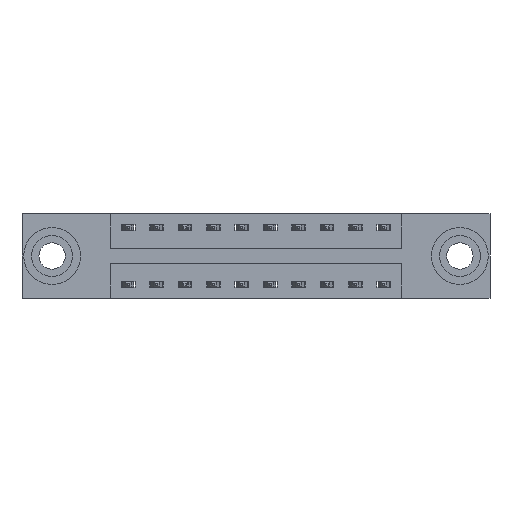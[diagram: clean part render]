
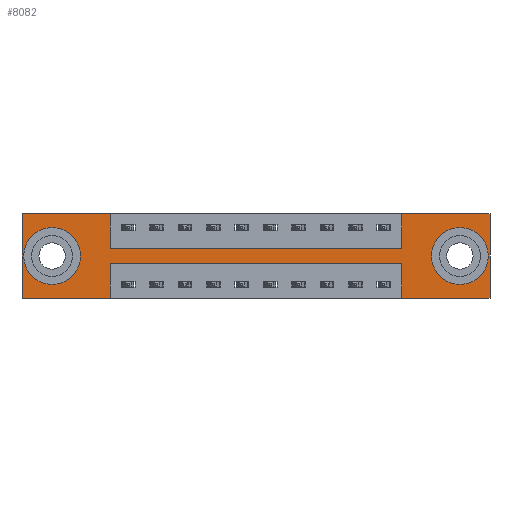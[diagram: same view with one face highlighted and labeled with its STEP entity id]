
A CAD part, front view. The second image highlights one B-rep face of the part: STEP entity #8082.
In plain terms, the highlighted planar face has unit normal (0, -1, 0).
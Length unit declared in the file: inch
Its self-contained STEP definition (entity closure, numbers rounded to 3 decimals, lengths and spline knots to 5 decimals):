
#42 = DIRECTION ( 'NONE',  ( 0., -1., 0. ) ) ;
#43 = FACE_BOUND ( 'NONE', #593, .T. ) ;
#147 = VECTOR ( 'NONE', #8115, 39.37008 ) ;
#241 = VERTEX_POINT ( 'NONE', #6588 ) ;
#277 = LINE ( 'NONE', #2341, #9574 ) ;
#318 = ORIENTED_EDGE ( 'NONE', *, *, #9186, .F. ) ;
#549 = LINE ( 'NONE', #3634, #4817 ) ;
#587 = CARTESIAN_POINT ( 'NONE',  ( 0.1325, 0., -0.107 ) ) ;
#593 = EDGE_LOOP ( 'NONE', ( #3263, #9373 ) ) ;
#647 = VERTEX_POINT ( 'NONE', #587 ) ;
#715 = ORIENTED_EDGE ( 'NONE', *, *, #3918, .F. ) ;
#737 = EDGE_CURVE ( 'NONE', #647, #7364, #2487, .T. ) ;
#756 = CARTESIAN_POINT ( 'NONE',  ( 2.06, 0., 0. ) ) ;
#1233 = ORIENTED_EDGE ( 'NONE', *, *, #1397, .F. ) ;
#1290 = VECTOR ( 'NONE', #8873, 39.37008 ) ;
#1392 = CARTESIAN_POINT ( 'NONE',  ( 1.9275, 0., -0.185 ) ) ;
#1397 = EDGE_CURVE ( 'NONE', #10675, #7529, #8215, .T. ) ;
#1768 = LINE ( 'NONE', #4602, #6515 ) ;
#1775 = VERTEX_POINT ( 'NONE', #10320 ) ;
#1825 = CARTESIAN_POINT ( 'NONE',  ( 0.1325, 0., -0.263 ) ) ;
#1854 = DIRECTION ( 'NONE',  ( 0., 0., -1. ) ) ;
#1980 = VECTOR ( 'NONE', #3044, 39.37008 ) ;
#1993 = EDGE_CURVE ( 'NONE', #7529, #5907, #9125, .T. ) ;
#2018 = CARTESIAN_POINT ( 'NONE',  ( 1.6725, 0., 0. ) ) ;
#2274 = DIRECTION ( 'NONE',  ( 0., 0., -1. ) ) ;
#2341 = CARTESIAN_POINT ( 'NONE',  ( 1.6725, 0., -0.37 ) ) ;
#2402 = VERTEX_POINT ( 'NONE', #4442 ) ;
#2419 = DIRECTION ( 'NONE',  ( 1., 0., 0. ) ) ;
#2438 = ORIENTED_EDGE ( 'NONE', *, *, #6224, .F. ) ;
#2453 = AXIS2_PLACEMENT_3D ( 'NONE', #4191, #8225, #9523 ) ;
#2487 = CIRCLE ( 'NONE', #2453, 0.078 ) ;
#2491 = DIRECTION ( 'NONE',  ( 0., 1., 0. ) ) ;
#2676 = CARTESIAN_POINT ( 'NONE',  ( 0.3875, 0., -0.22 ) ) ;
#2740 = CARTESIAN_POINT ( 'NONE',  ( 0., 0., -0.37 ) ) ;
#2778 = DIRECTION ( 'NONE',  ( 1., 0., 0. ) ) ;
#3044 = DIRECTION ( 'NONE',  ( -1., 0., 0. ) ) ;
#3046 = VERTEX_POINT ( 'NONE', #3427 ) ;
#3263 = ORIENTED_EDGE ( 'NONE', *, *, #737, .T. ) ;
#3427 = CARTESIAN_POINT ( 'NONE',  ( 1.6725, 0., -0.22 ) ) ;
#3443 = CARTESIAN_POINT ( 'NONE',  ( 1.9275, 0., -0.185 ) ) ;
#3548 = EDGE_CURVE ( 'NONE', #7974, #2402, #10690, .T. ) ;
#3634 = CARTESIAN_POINT ( 'NONE',  ( 0.3875, 0., 0. ) ) ;
#3750 = EDGE_CURVE ( 'NONE', #7364, #647, #6431, .T. ) ;
#3839 = VERTEX_POINT ( 'NONE', #7047 ) ;
#3918 = EDGE_CURVE ( 'NONE', #5907, #3839, #9751, .T. ) ;
#3941 = LINE ( 'NONE', #9022, #8484 ) ;
#3961 = CIRCLE ( 'NONE', #11416, 0.078 ) ;
#4191 = CARTESIAN_POINT ( 'NONE',  ( 0.1325, 0., -0.185 ) ) ;
#4267 = CARTESIAN_POINT ( 'NONE',  ( 0.3875, 0., -0.22 ) ) ;
#4363 = DIRECTION ( 'NONE',  ( 0., 0., -1. ) ) ;
#4442 = CARTESIAN_POINT ( 'NONE',  ( 2.06, 0., -0.37 ) ) ;
#4578 = FACE_OUTER_BOUND ( 'NONE', #4619, .T. ) ;
#4602 = CARTESIAN_POINT ( 'NONE',  ( 0.3875, 0., -0.15 ) ) ;
#4619 = EDGE_LOOP ( 'NONE', ( #1233, #8250, #318, #7291, #11129, #2438, #9044, #7081, #7848, #4879, #715, #5430 ) ) ;
#4711 = VERTEX_POINT ( 'NONE', #5463 ) ;
#4817 = VECTOR ( 'NONE', #1854, 39.37008 ) ;
#4828 = CARTESIAN_POINT ( 'NONE',  ( 0.3875, 0., -0.37 ) ) ;
#4838 = VERTEX_POINT ( 'NONE', #2018 ) ;
#4879 = ORIENTED_EDGE ( 'NONE', *, *, #10618, .F. ) ;
#4965 = LINE ( 'NONE', #2676, #147 ) ;
#5098 = VECTOR ( 'NONE', #10049, 39.37008 ) ;
#5238 = LINE ( 'NONE', #6899, #7070 ) ;
#5394 = VERTEX_POINT ( 'NONE', #7698 ) ;
#5430 = ORIENTED_EDGE ( 'NONE', *, *, #1993, .F. ) ;
#5449 = VECTOR ( 'NONE', #11094, 39.37008 ) ;
#5463 = CARTESIAN_POINT ( 'NONE',  ( 0.3875, 0., 0. ) ) ;
#5465 = PLANE ( 'NONE',  #10053 ) ;
#5556 = EDGE_CURVE ( 'NONE', #8722, #1775, #5684, .T. ) ;
#5628 = CARTESIAN_POINT ( 'NONE',  ( 1.6725, 0., 0. ) ) ;
#5684 = CIRCLE ( 'NONE', #10888, 0.078 ) ;
#5907 = VERTEX_POINT ( 'NONE', #9431 ) ;
#5932 = VERTEX_POINT ( 'NONE', #11210 ) ;
#6224 = EDGE_CURVE ( 'NONE', #4838, #7974, #8787, .T. ) ;
#6352 = CARTESIAN_POINT ( 'NONE',  ( 0., 0., 0. ) ) ;
#6366 = DIRECTION ( 'NONE',  ( 0., 0., -1. ) ) ;
#6388 = VECTOR ( 'NONE', #9053, 39.37008 ) ;
#6431 = CIRCLE ( 'NONE', #8530, 0.078 ) ;
#6515 = VECTOR ( 'NONE', #2778, 39.37008 ) ;
#6588 = CARTESIAN_POINT ( 'NONE',  ( 1.6725, 0., -0.37 ) ) ;
#6788 = EDGE_CURVE ( 'NONE', #3046, #10675, #4965, .T. ) ;
#6899 = CARTESIAN_POINT ( 'NONE',  ( 0., 0., 0. ) ) ;
#7047 = CARTESIAN_POINT ( 'NONE',  ( 0., 0., 0. ) ) ;
#7070 = VECTOR ( 'NONE', #2419, 39.37008 ) ;
#7081 = ORIENTED_EDGE ( 'NONE', *, *, #10315, .F. ) ;
#7128 = CARTESIAN_POINT ( 'NONE',  ( 0., 0., 0. ) ) ;
#7131 = VECTOR ( 'NONE', #8071, 39.37008 ) ;
#7291 = ORIENTED_EDGE ( 'NONE', *, *, #7407, .F. ) ;
#7364 = VERTEX_POINT ( 'NONE', #1825 ) ;
#7407 = EDGE_CURVE ( 'NONE', #2402, #241, #3941, .T. ) ;
#7529 = VERTEX_POINT ( 'NONE', #4828 ) ;
#7687 = DIRECTION ( 'NONE',  ( 0., 1., 0. ) ) ;
#7698 = CARTESIAN_POINT ( 'NONE',  ( 1.6725, 0., -0.15 ) ) ;
#7848 = ORIENTED_EDGE ( 'NONE', *, *, #10905, .F. ) ;
#7908 = CARTESIAN_POINT ( 'NONE',  ( 0.1325, 0., -0.185 ) ) ;
#7974 = VERTEX_POINT ( 'NONE', #756 ) ;
#8071 = DIRECTION ( 'NONE',  ( 0., 0., 1. ) ) ;
#8082 = ADVANCED_FACE ( 'NONE', ( #9070, #43, #4578 ), #5465, .T. ) ;
#8115 = DIRECTION ( 'NONE',  ( -1., 0., 0. ) ) ;
#8215 = LINE ( 'NONE', #8791, #1290 ) ;
#8225 = DIRECTION ( 'NONE',  ( 0., 1., 0. ) ) ;
#8250 = ORIENTED_EDGE ( 'NONE', *, *, #6788, .F. ) ;
#8484 = VECTOR ( 'NONE', #10736, 39.37008 ) ;
#8530 = AXIS2_PLACEMENT_3D ( 'NONE', #7908, #2491, #8790 ) ;
#8638 = DIRECTION ( 'NONE',  ( 0., 0., 1. ) ) ;
#8722 = VERTEX_POINT ( 'NONE', #9880 ) ;
#8787 = LINE ( 'NONE', #6352, #6388 ) ;
#8790 = DIRECTION ( 'NONE',  ( 0., 0., 1. ) ) ;
#8791 = CARTESIAN_POINT ( 'NONE',  ( 0.3875, 0., -0.37 ) ) ;
#8873 = DIRECTION ( 'NONE',  ( 0., 0., -1. ) ) ;
#8937 = ORIENTED_EDGE ( 'NONE', *, *, #5556, .T. ) ;
#9022 = CARTESIAN_POINT ( 'NONE',  ( 0., 0., -0.37 ) ) ;
#9044 = ORIENTED_EDGE ( 'NONE', *, *, #9755, .F. ) ;
#9053 = DIRECTION ( 'NONE',  ( 1., 0., 0. ) ) ;
#9070 = FACE_BOUND ( 'NONE', #9570, .T. ) ;
#9125 = LINE ( 'NONE', #11004, #1980 ) ;
#9186 = EDGE_CURVE ( 'NONE', #241, #3046, #277, .T. ) ;
#9373 = ORIENTED_EDGE ( 'NONE', *, *, #3750, .T. ) ;
#9384 = CARTESIAN_POINT ( 'NONE',  ( 2.06, 0., 0. ) ) ;
#9431 = CARTESIAN_POINT ( 'NONE',  ( 0., 0., -0.37 ) ) ;
#9523 = DIRECTION ( 'NONE',  ( 0., 0., 1. ) ) ;
#9570 = EDGE_LOOP ( 'NONE', ( #11211, #8937 ) ) ;
#9574 = VECTOR ( 'NONE', #8638, 39.37008 ) ;
#9698 = DIRECTION ( 'NONE',  ( 0., 1., 0. ) ) ;
#9751 = LINE ( 'NONE', #7128, #7131 ) ;
#9755 = EDGE_CURVE ( 'NONE', #5394, #4838, #9830, .T. ) ;
#9830 = LINE ( 'NONE', #5628, #5098 ) ;
#9880 = CARTESIAN_POINT ( 'NONE',  ( 1.9275, 0., -0.263 ) ) ;
#10049 = DIRECTION ( 'NONE',  ( 0., 0., 1. ) ) ;
#10053 = AXIS2_PLACEMENT_3D ( 'NONE', #2740, #42, #6366 ) ;
#10315 = EDGE_CURVE ( 'NONE', #5932, #5394, #1768, .T. ) ;
#10320 = CARTESIAN_POINT ( 'NONE',  ( 1.9275, 0., -0.107 ) ) ;
#10534 = EDGE_CURVE ( 'NONE', #1775, #8722, #3961, .T. ) ;
#10618 = EDGE_CURVE ( 'NONE', #3839, #4711, #5238, .T. ) ;
#10675 = VERTEX_POINT ( 'NONE', #4267 ) ;
#10690 = LINE ( 'NONE', #9384, #5449 ) ;
#10736 = DIRECTION ( 'NONE',  ( -1., 0., 0. ) ) ;
#10888 = AXIS2_PLACEMENT_3D ( 'NONE', #3443, #9698, #4363 ) ;
#10905 = EDGE_CURVE ( 'NONE', #4711, #5932, #549, .T. ) ;
#11004 = CARTESIAN_POINT ( 'NONE',  ( 0., 0., -0.37 ) ) ;
#11094 = DIRECTION ( 'NONE',  ( 0., 0., -1. ) ) ;
#11129 = ORIENTED_EDGE ( 'NONE', *, *, #3548, .F. ) ;
#11210 = CARTESIAN_POINT ( 'NONE',  ( 0.3875, 0., -0.15 ) ) ;
#11211 = ORIENTED_EDGE ( 'NONE', *, *, #10534, .T. ) ;
#11416 = AXIS2_PLACEMENT_3D ( 'NONE', #1392, #7687, #2274 ) ;
